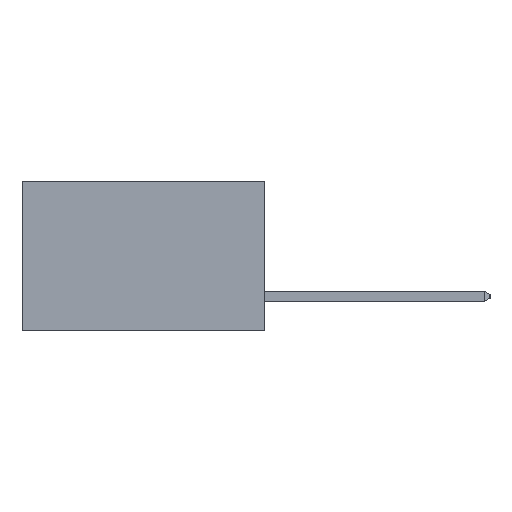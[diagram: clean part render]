
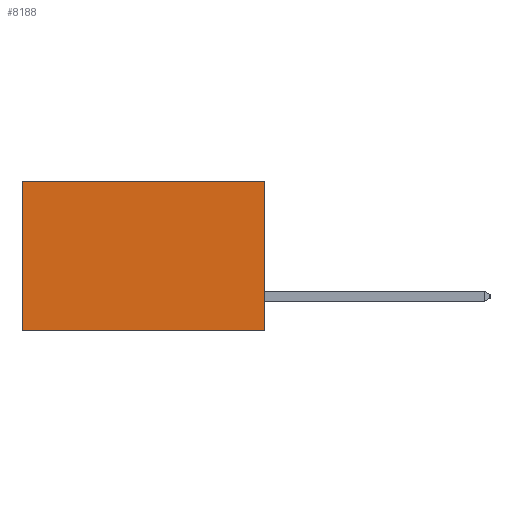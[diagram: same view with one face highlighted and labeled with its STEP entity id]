
A CAD part, left-side view. The second image highlights one B-rep face of the part: STEP entity #8188.
In plain terms, the highlighted planar face has unit normal (-1, 0, 0).
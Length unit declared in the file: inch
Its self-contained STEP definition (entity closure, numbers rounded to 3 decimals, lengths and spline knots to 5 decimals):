
#48 = LINE ( 'NONE', #10313, #6008 ) ;
#363 = CARTESIAN_POINT ( 'NONE',  ( 0.2615, 0., -0.37 ) ) ;
#1364 = VERTEX_POINT ( 'NONE', #17130 ) ;
#1467 = LINE ( 'NONE', #14661, #12138 ) ;
#3199 = CARTESIAN_POINT ( 'NONE',  ( 0.2615, 0.6, -0.37 ) ) ;
#3408 = VECTOR ( 'NONE', #11180, 39.37008 ) ;
#4473 = DIRECTION ( 'NONE',  ( 0., 0., -1. ) ) ;
#4482 = VERTEX_POINT ( 'NONE', #10685 ) ;
#4679 = ORIENTED_EDGE ( 'NONE', *, *, #6794, .F. ) ;
#6008 = VECTOR ( 'NONE', #7707, 39.37008 ) ;
#6281 = EDGE_CURVE ( 'NONE', #4482, #12164, #1467, .T. ) ;
#6794 = EDGE_CURVE ( 'NONE', #4482, #1364, #7350, .T. ) ;
#6961 = LINE ( 'NONE', #3199, #3408 ) ;
#6988 = ORIENTED_EDGE ( 'NONE', *, *, #11258, .T. ) ;
#7344 = AXIS2_PLACEMENT_3D ( 'NONE', #363, #12464, #4473 ) ;
#7350 = LINE ( 'NONE', #10717, #16996 ) ;
#7707 = DIRECTION ( 'NONE',  ( 0., 1., 0. ) ) ;
#8188 = ADVANCED_FACE ( 'NONE', ( #12271 ), #13716, .F. ) ;
#10313 = CARTESIAN_POINT ( 'NONE',  ( 0.2615, 0., -0.37 ) ) ;
#10682 = DIRECTION ( 'NONE',  ( 0., 0., -1. ) ) ;
#10685 = CARTESIAN_POINT ( 'NONE',  ( 0.2615, 0., 0. ) ) ;
#10717 = CARTESIAN_POINT ( 'NONE',  ( 0.2615, 0., -0.37 ) ) ;
#11180 = DIRECTION ( 'NONE',  ( 0., 0., -1. ) ) ;
#11258 = EDGE_CURVE ( 'NONE', #12164, #11343, #6961, .T. ) ;
#11343 = VERTEX_POINT ( 'NONE', #15284 ) ;
#12138 = VECTOR ( 'NONE', #14774, 39.37008 ) ;
#12164 = VERTEX_POINT ( 'NONE', #15725 ) ;
#12271 = FACE_OUTER_BOUND ( 'NONE', #16275, .T. ) ;
#12464 = DIRECTION ( 'NONE',  ( 1., 0., 0. ) ) ;
#13716 = PLANE ( 'NONE',  #7344 ) ;
#14661 = CARTESIAN_POINT ( 'NONE',  ( 0.2615, 0., 0. ) ) ;
#14774 = DIRECTION ( 'NONE',  ( 0., 1., 0. ) ) ;
#15256 = ORIENTED_EDGE ( 'NONE', *, *, #6281, .T. ) ;
#15284 = CARTESIAN_POINT ( 'NONE',  ( 0.2615, 0.6, -0.37 ) ) ;
#15725 = CARTESIAN_POINT ( 'NONE',  ( 0.2615, 0.6, 0. ) ) ;
#16105 = ORIENTED_EDGE ( 'NONE', *, *, #16736, .F. ) ;
#16275 = EDGE_LOOP ( 'NONE', ( #6988, #16105, #4679, #15256 ) ) ;
#16736 = EDGE_CURVE ( 'NONE', #1364, #11343, #48, .T. ) ;
#16996 = VECTOR ( 'NONE', #10682, 39.37008 ) ;
#17130 = CARTESIAN_POINT ( 'NONE',  ( 0.2615, 0., -0.37 ) ) ;
